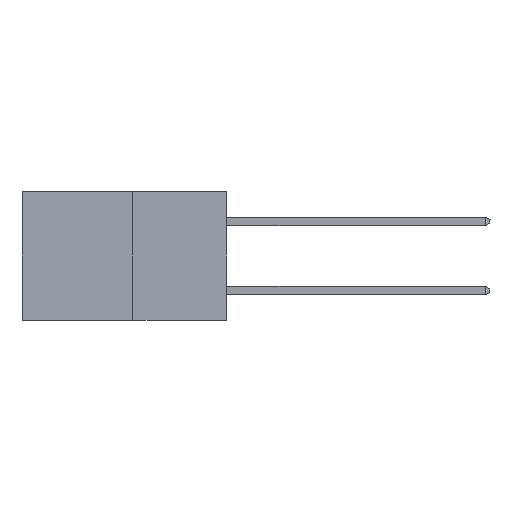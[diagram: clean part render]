
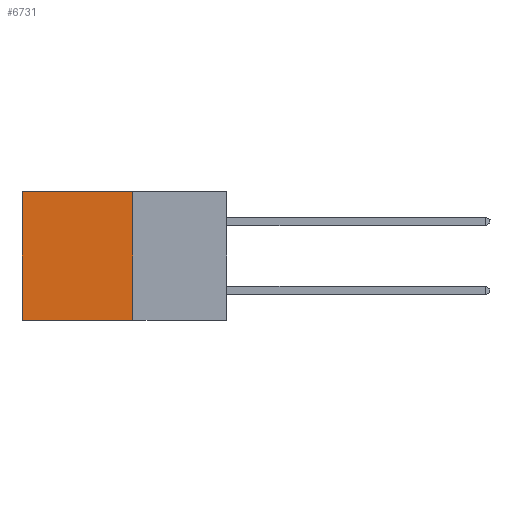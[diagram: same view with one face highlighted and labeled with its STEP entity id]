
A CAD part, left-side view. The second image highlights one B-rep face of the part: STEP entity #6731.
In plain terms, the highlighted planar face has unit normal (-1, 0, 0).
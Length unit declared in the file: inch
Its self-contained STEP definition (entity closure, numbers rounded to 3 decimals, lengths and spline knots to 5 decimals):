
#373 = VECTOR ( 'NONE', #7300, 39.37008 ) ;
#1722 = ORIENTED_EDGE ( 'NONE', *, *, #5435, .F. ) ;
#2304 = LINE ( 'NONE', #11071, #11820 ) ;
#2613 = LINE ( 'NONE', #4512, #12326 ) ;
#3397 = DIRECTION ( 'NONE',  ( 0., 0., -1. ) ) ;
#3588 = VERTEX_POINT ( 'NONE', #9831 ) ;
#4512 = CARTESIAN_POINT ( 'NONE',  ( 0.277, 0.59, -0.37 ) ) ;
#4610 = CARTESIAN_POINT ( 'NONE',  ( 0.277, 0.59, -0.37 ) ) ;
#4827 = VERTEX_POINT ( 'NONE', #10839 ) ;
#5020 = ORIENTED_EDGE ( 'NONE', *, *, #9380, .T. ) ;
#5435 = EDGE_CURVE ( 'NONE', #6745, #6679, #10086, .T. ) ;
#6033 = ORIENTED_EDGE ( 'NONE', *, *, #8745, .T. ) ;
#6077 = CARTESIAN_POINT ( 'NONE',  ( 0.277, 0.27, 0. ) ) ;
#6112 = DIRECTION ( 'NONE',  ( 0., 1., 0. ) ) ;
#6679 = VERTEX_POINT ( 'NONE', #4610 ) ;
#6731 = ADVANCED_FACE ( 'NONE', ( #6932 ), #8119, .F. ) ;
#6745 = VERTEX_POINT ( 'NONE', #8824 ) ;
#6932 = FACE_OUTER_BOUND ( 'NONE', #12297, .T. ) ;
#7300 = DIRECTION ( 'NONE',  ( 0., 1., 0. ) ) ;
#7743 = EDGE_CURVE ( 'NONE', #3588, #6745, #2304, .T. ) ;
#8099 = DIRECTION ( 'NONE',  ( 1., 0., 0. ) ) ;
#8119 = PLANE ( 'NONE',  #8201 ) ;
#8201 = AXIS2_PLACEMENT_3D ( 'NONE', #8980, #8099, #12254 ) ;
#8745 = EDGE_CURVE ( 'NONE', #4827, #6679, #2613, .T. ) ;
#8824 = CARTESIAN_POINT ( 'NONE',  ( 0.277, 0.27, -0.37 ) ) ;
#8980 = CARTESIAN_POINT ( 'NONE',  ( 0.277, 0.27, -0.37 ) ) ;
#9380 = EDGE_CURVE ( 'NONE', #3588, #4827, #9953, .T. ) ;
#9670 = VECTOR ( 'NONE', #6112, 39.37008 ) ;
#9831 = CARTESIAN_POINT ( 'NONE',  ( 0.277, 0.27, 0. ) ) ;
#9953 = LINE ( 'NONE', #6077, #9670 ) ;
#10086 = LINE ( 'NONE', #10474, #373 ) ;
#10474 = CARTESIAN_POINT ( 'NONE',  ( 0.277, 0.27, -0.37 ) ) ;
#10839 = CARTESIAN_POINT ( 'NONE',  ( 0.277, 0.59, 0. ) ) ;
#11071 = CARTESIAN_POINT ( 'NONE',  ( 0.277, 0.27, -0.37 ) ) ;
#11143 = DIRECTION ( 'NONE',  ( 0., 0., -1. ) ) ;
#11328 = ORIENTED_EDGE ( 'NONE', *, *, #7743, .F. ) ;
#11820 = VECTOR ( 'NONE', #11143, 39.37008 ) ;
#12254 = DIRECTION ( 'NONE',  ( 0., 0., -1. ) ) ;
#12297 = EDGE_LOOP ( 'NONE', ( #6033, #1722, #11328, #5020 ) ) ;
#12326 = VECTOR ( 'NONE', #3397, 39.37008 ) ;
